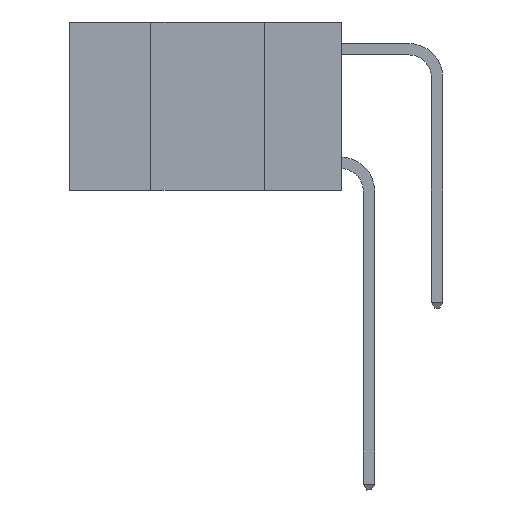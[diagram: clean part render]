
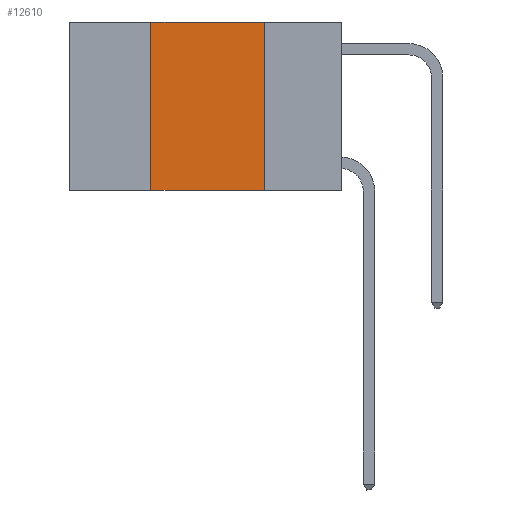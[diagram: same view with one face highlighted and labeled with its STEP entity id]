
A CAD part, left-side view. The second image highlights one B-rep face of the part: STEP entity #12610.
In plain terms, the highlighted planar face has unit normal (-1, 0, 0).
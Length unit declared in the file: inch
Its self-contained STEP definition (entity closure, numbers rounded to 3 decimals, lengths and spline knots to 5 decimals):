
#53 = ORIENTED_EDGE ( 'NONE', *, *, #1040, .F. ) ;
#747 = LINE ( 'NONE', #12203, #12607 ) ;
#809 = DIRECTION ( 'NONE',  ( 0., 0., -1. ) ) ;
#1040 = EDGE_CURVE ( 'NONE', #9555, #21326, #20583, .T. ) ;
#1375 = ORIENTED_EDGE ( 'NONE', *, *, #20657, .F. ) ;
#1816 = DIRECTION ( 'NONE',  ( 0., 0., -1. ) ) ;
#2109 = VECTOR ( 'NONE', #19625, 39.37008 ) ;
#2339 = EDGE_CURVE ( 'NONE', #9555, #19980, #747, .T. ) ;
#2817 = VECTOR ( 'NONE', #809, 39.37008 ) ;
#3585 = PLANE ( 'NONE',  #6092 ) ;
#3820 = DIRECTION ( 'NONE',  ( 0., 0., 1. ) ) ;
#4323 = CARTESIAN_POINT ( 'NONE',  ( 0., 0.6, 0. ) ) ;
#5475 = CARTESIAN_POINT ( 'NONE',  ( 0., 0.42, 0. ) ) ;
#6092 = AXIS2_PLACEMENT_3D ( 'NONE', #20224, #8547, #1816 ) ;
#7340 = EDGE_CURVE ( 'NONE', #9599, #19980, #17539, .T. ) ;
#8547 = DIRECTION ( 'NONE',  ( 1., 0., 0. ) ) ;
#9020 = ORIENTED_EDGE ( 'NONE', *, *, #7340, .F. ) ;
#9555 = VERTEX_POINT ( 'NONE', #15562 ) ;
#9583 = CARTESIAN_POINT ( 'NONE',  ( 0., 0.17, -0.37 ) ) ;
#9599 = VERTEX_POINT ( 'NONE', #15670 ) ;
#10292 = CARTESIAN_POINT ( 'NONE',  ( 0., 0.42, 0. ) ) ;
#12203 = CARTESIAN_POINT ( 'NONE',  ( 0., 0.6, -0.37 ) ) ;
#12607 = VECTOR ( 'NONE', #21015, 39.37008 ) ;
#12610 = ADVANCED_FACE ( 'NONE', ( #18671 ), #3585, .F. ) ;
#13766 = ORIENTED_EDGE ( 'NONE', *, *, #2339, .T. ) ;
#15562 = CARTESIAN_POINT ( 'NONE',  ( 0., 0.42, -0.37 ) ) ;
#15670 = CARTESIAN_POINT ( 'NONE',  ( 0., 0.17, 0. ) ) ;
#16116 = LINE ( 'NONE', #4323, #2109 ) ;
#17003 = EDGE_LOOP ( 'NONE', ( #9020, #1375, #53, #13766 ) ) ;
#17539 = LINE ( 'NONE', #21065, #2817 ) ;
#17822 = VECTOR ( 'NONE', #3820, 39.37008 ) ;
#18671 = FACE_OUTER_BOUND ( 'NONE', #17003, .T. ) ;
#19625 = DIRECTION ( 'NONE',  ( 0., -1., 0. ) ) ;
#19980 = VERTEX_POINT ( 'NONE', #9583 ) ;
#20224 = CARTESIAN_POINT ( 'NONE',  ( 0., 0.6, 0. ) ) ;
#20583 = LINE ( 'NONE', #5475, #17822 ) ;
#20657 = EDGE_CURVE ( 'NONE', #21326, #9599, #16116, .T. ) ;
#21015 = DIRECTION ( 'NONE',  ( 0., -1., 0. ) ) ;
#21065 = CARTESIAN_POINT ( 'NONE',  ( 0., 0.17, 0. ) ) ;
#21326 = VERTEX_POINT ( 'NONE', #10292 ) ;
